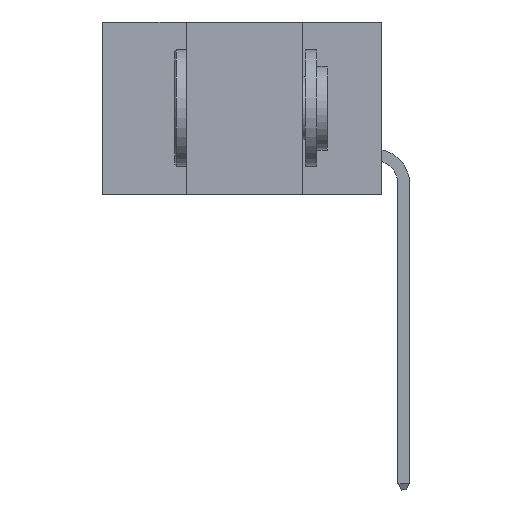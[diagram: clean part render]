
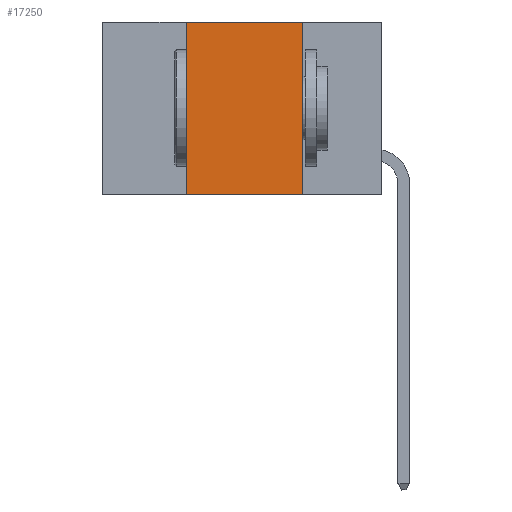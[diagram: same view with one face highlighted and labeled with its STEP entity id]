
A CAD part, left-side view. The second image highlights one B-rep face of the part: STEP entity #17250.
In plain terms, the highlighted planar face has unit normal (-1, 0, 0).
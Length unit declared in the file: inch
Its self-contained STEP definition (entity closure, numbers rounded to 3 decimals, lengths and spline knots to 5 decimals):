
#944 = DIRECTION ( 'NONE',  ( 0., -1., 0. ) ) ;
#1548 = PLANE ( 'NONE',  #15266 ) ;
#2333 = CARTESIAN_POINT ( 'NONE',  ( 0., 0.42, -0.37 ) ) ;
#2688 = DIRECTION ( 'NONE',  ( 0., 0., 1. ) ) ;
#3435 = EDGE_CURVE ( 'NONE', #21852, #19659, #8994, .T. ) ;
#5761 = LINE ( 'NONE', #12712, #27143 ) ;
#5970 = CARTESIAN_POINT ( 'NONE',  ( 0., 0.17, -0.37 ) ) ;
#6442 = ORIENTED_EDGE ( 'NONE', *, *, #11299, .F. ) ;
#6915 = LINE ( 'NONE', #21925, #25347 ) ;
#7862 = CARTESIAN_POINT ( 'NONE',  ( 0., 0.17, 0. ) ) ;
#8490 = DIRECTION ( 'NONE',  ( 1., 0., 0. ) ) ;
#8994 = LINE ( 'NONE', #21001, #12700 ) ;
#11299 = EDGE_CURVE ( 'NONE', #21852, #18818, #6915, .T. ) ;
#12700 = VECTOR ( 'NONE', #23055, 39.37008 ) ;
#12712 = CARTESIAN_POINT ( 'NONE',  ( 0., 0.17, 0. ) ) ;
#12954 = ORIENTED_EDGE ( 'NONE', *, *, #27805, .F. ) ;
#13334 = CARTESIAN_POINT ( 'NONE',  ( 0., 0.6, 0. ) ) ;
#14167 = EDGE_LOOP ( 'NONE', ( #12954, #20811, #6442, #27102 ) ) ;
#15124 = CARTESIAN_POINT ( 'NONE',  ( 0., 0.6, 0. ) ) ;
#15229 = FACE_OUTER_BOUND ( 'NONE', #14167, .T. ) ;
#15266 = AXIS2_PLACEMENT_3D ( 'NONE', #13334, #8490, #27554 ) ;
#17250 = ADVANCED_FACE ( 'NONE', ( #15229 ), #1548, .F. ) ;
#17662 = VERTEX_POINT ( 'NONE', #7862 ) ;
#18818 = VERTEX_POINT ( 'NONE', #28793 ) ;
#19088 = EDGE_CURVE ( 'NONE', #18818, #17662, #29321, .T. ) ;
#19659 = VERTEX_POINT ( 'NONE', #5970 ) ;
#20811 = ORIENTED_EDGE ( 'NONE', *, *, #19088, .F. ) ;
#21001 = CARTESIAN_POINT ( 'NONE',  ( 0., 0.6, -0.37 ) ) ;
#21852 = VERTEX_POINT ( 'NONE', #2333 ) ;
#21925 = CARTESIAN_POINT ( 'NONE',  ( 0., 0.42, 0. ) ) ;
#22220 = DIRECTION ( 'NONE',  ( 0., 0., -1. ) ) ;
#23055 = DIRECTION ( 'NONE',  ( 0., -1., 0. ) ) ;
#25347 = VECTOR ( 'NONE', #2688, 39.37008 ) ;
#26345 = VECTOR ( 'NONE', #944, 39.37008 ) ;
#27102 = ORIENTED_EDGE ( 'NONE', *, *, #3435, .T. ) ;
#27143 = VECTOR ( 'NONE', #22220, 39.37008 ) ;
#27554 = DIRECTION ( 'NONE',  ( 0., 0., -1. ) ) ;
#27805 = EDGE_CURVE ( 'NONE', #17662, #19659, #5761, .T. ) ;
#28793 = CARTESIAN_POINT ( 'NONE',  ( 0., 0.42, 0. ) ) ;
#29321 = LINE ( 'NONE', #15124, #26345 ) ;
